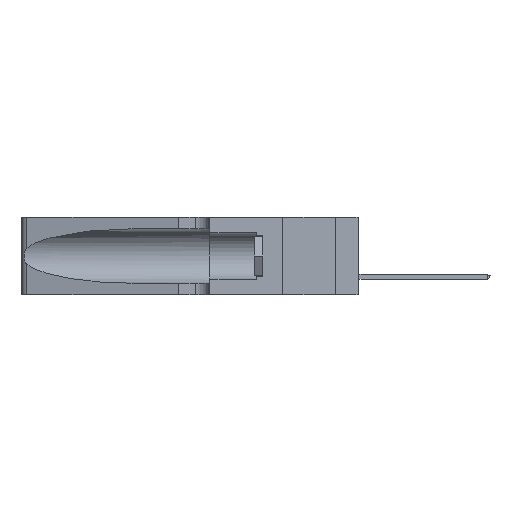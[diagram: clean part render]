
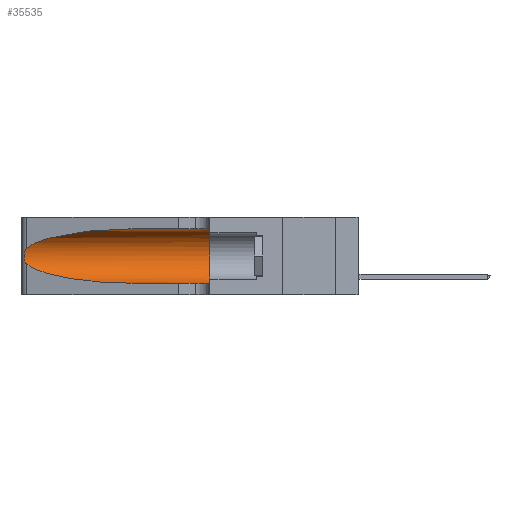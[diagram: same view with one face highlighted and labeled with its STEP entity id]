
A CAD part, left-side view. The second image highlights one B-rep face of the part: STEP entity #35535.
In plain terms, the highlighted cylindrical face has radius 3.308 mm (diameter 6.617 mm), a partial arc.
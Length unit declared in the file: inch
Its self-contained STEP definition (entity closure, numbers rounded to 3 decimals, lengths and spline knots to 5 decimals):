
#2345 = CARTESIAN_POINT ( 'NONE',  ( 0.1305, 0.72297, 0.05475 ) ) ;
#2667 = ORIENTED_EDGE ( 'NONE', *, *, #5160, .T. ) ;
#2709 = AXIS2_PLACEMENT_3D ( 'NONE', #33902, #11928, #28743 ) ;
#3378 = EDGE_LOOP ( 'NONE', ( #2667, #14993, #24889, #30679, #30256, #20336 ) ) ;
#3844 = CARTESIAN_POINT ( 'NONE',  ( 0.25487, 1.22718, 0.22369 ) ) ;
#3868 = CARTESIAN_POINT ( 'NONE',  ( 0.2373, 1.15595, 0.28018 ) ) ;
#4528 = VERTEX_POINT ( 'NONE', #35664 ) ;
#5133 = CARTESIAN_POINT ( 'NONE',  ( 0.1305, 0.72297, 0.31525 ) ) ;
#5160 = EDGE_CURVE ( 'NONE', #8227, #20518, #6681, .T. ) ;
#5359 = CARTESIAN_POINT ( 'NONE',  ( 0.1305, 0.35, 0.185 ) ) ;
#6681 =( BOUNDED_CURVE ( )  B_SPLINE_CURVE ( 3, ( #5133, #31014, #3868, #28514 ),
 .UNSPECIFIED., .F., .T. ) 
 B_SPLINE_CURVE_WITH_KNOTS ( ( 4, 4 ),
 ( 1.5708, 2.84003 ),
 .UNSPECIFIED. ) 
 CURVE ( )  GEOMETRIC_REPRESENTATION_ITEM ( )  RATIONAL_B_SPLINE_CURVE ( ( 1., 0.87, 0.87, 1. ) ) 
 REPRESENTATION_ITEM ( '' )  );
#7205 = CARTESIAN_POINT ( 'NONE',  ( 0.25639, 1.23184, 0.21858 ) ) ;
#7455 = CARTESIAN_POINT ( 'NONE',  ( 0.25487, 1.22718, 0.14631 ) ) ;
#7989 = CARTESIAN_POINT ( 'NONE',  ( 0.18966, 0.96281, 0.05475 ) ) ;
#8227 = VERTEX_POINT ( 'NONE', #12474 ) ;
#9101 = EDGE_CURVE ( 'NONE', #24137, #17811, #9318, .T. ) ;
#9318 =( BOUNDED_CURVE ( )  B_SPLINE_CURVE ( 3, ( #13550, #18970, #7989, #2345 ),
 .UNSPECIFIED., .F., .F. ) 
 B_SPLINE_CURVE_WITH_KNOTS ( ( 4, 4 ),
 ( 3.44316, 4.71239 ),
 .UNSPECIFIED. ) 
 CURVE ( )  GEOMETRIC_REPRESENTATION_ITEM ( )  RATIONAL_B_SPLINE_CURVE ( ( 1., 0.87, 0.87, 1. ) ) 
 REPRESENTATION_ITEM ( '' )  );
#9974 = CARTESIAN_POINT ( 'NONE',  ( 0.25789, 1.23486, 0.15765 ) ) ;
#11136 = AXIS2_PLACEMENT_3D ( 'NONE', #5359, #24618, #32941 ) ;
#11262 = CARTESIAN_POINT ( 'NONE',  ( 0.1305, 1.61858, 0.31525 ) ) ;
#11928 = DIRECTION ( 'NONE',  ( 0., -1., 0. ) ) ;
#12474 = CARTESIAN_POINT ( 'NONE',  ( 0.1305, 0.72297, 0.31525 ) ) ;
#13550 = CARTESIAN_POINT ( 'NONE',  ( 0.25487, 1.22718, 0.14631 ) ) ;
#14307 = FACE_OUTER_BOUND ( 'NONE', #3378, .T. ) ;
#14993 = ORIENTED_EDGE ( 'NONE', *, *, #34136, .T. ) ;
#15282 = CARTESIAN_POINT ( 'NONE',  ( 0.25787, 1.23484, 0.2124 ) ) ;
#15408 = CARTESIAN_POINT ( 'NONE',  ( 0.26075, 1.23896, 0.178 ) ) ;
#16091 = EDGE_CURVE ( 'NONE', #4528, #29876, #18589, .T. ) ;
#16310 = CARTESIAN_POINT ( 'NONE',  ( 0.25487, 1.22718, 0.14631 ) ) ;
#17081 = LINE ( 'NONE', #22098, #18355 ) ;
#17811 = VERTEX_POINT ( 'NONE', #28584 ) ;
#17942 = CARTESIAN_POINT ( 'NONE',  ( 0.25854, 1.2359, 0.20912 ) ) ;
#18355 = VECTOR ( 'NONE', #33048, 39.37008 ) ;
#18589 = CIRCLE ( 'NONE', #11136, 0.13025 ) ;
#18970 = CARTESIAN_POINT ( 'NONE',  ( 0.2373, 1.15595, 0.08982 ) ) ;
#19556 = VECTOR ( 'NONE', #19923, 39.37008 ) ;
#19923 = DIRECTION ( 'NONE',  ( 0., -1., 0. ) ) ;
#20336 = ORIENTED_EDGE ( 'NONE', *, *, #20964, .F. ) ;
#20518 = VERTEX_POINT ( 'NONE', #3844 ) ;
#20623 = CARTESIAN_POINT ( 'NONE',  ( 0.25555, 1.22994, 0.2215 ) ) ;
#20749 = CARTESIAN_POINT ( 'NONE',  ( 0.26018, 1.23835, 0.19895 ) ) ;
#20964 = EDGE_CURVE ( 'NONE', #8227, #4528, #31642, .T. ) ;
#20988 = CARTESIAN_POINT ( 'NONE',  ( 0.26017, 1.23833, 0.17102 ) ) ;
#22098 = CARTESIAN_POINT ( 'NONE',  ( 0.1305, 1.61858, 0.05475 ) ) ;
#22159 = CARTESIAN_POINT ( 'NONE',  ( 0.1305, 0.35, 0.05475 ) ) ;
#24137 = VERTEX_POINT ( 'NONE', #16310 ) ;
#24618 = DIRECTION ( 'NONE',  ( 0., 1., 0. ) ) ;
#24668 = CYLINDRICAL_SURFACE ( 'NONE', #2709, 0.13025 ) ;
#24889 = ORIENTED_EDGE ( 'NONE', *, *, #9101, .T. ) ;
#26338 = EDGE_CURVE ( 'NONE', #17811, #29876, #17081, .T. ) ;
#26525 = CARTESIAN_POINT ( 'NONE',  ( 0.25856, 1.23593, 0.16098 ) ) ;
#28514 = CARTESIAN_POINT ( 'NONE',  ( 0.25487, 1.22718, 0.22369 ) ) ;
#28584 = CARTESIAN_POINT ( 'NONE',  ( 0.1305, 0.72297, 0.05475 ) ) ;
#28743 = DIRECTION ( 'NONE',  ( 0., 0., -1. ) ) ;
#29876 = VERTEX_POINT ( 'NONE', #22159 ) ;
#30256 = ORIENTED_EDGE ( 'NONE', *, *, #16091, .F. ) ;
#30679 = ORIENTED_EDGE ( 'NONE', *, *, #26338, .T. ) ;
#31014 = CARTESIAN_POINT ( 'NONE',  ( 0.18966, 0.96281, 0.31525 ) ) ;
#31224 = B_SPLINE_CURVE_WITH_KNOTS ( 'NONE', 3,
 ( #31928, #20623, #7205, #15282, #17942, #20749, #31691, #15408, #20988, #26525, #9974, #32052, #32163, #7455 ),
 .UNSPECIFIED., .F., .F.,
 ( 4, 2, 2, 2, 2, 2, 4 ),
 ( 0., 0.00027, 0.00053, 0.00107, 0.0016, 0.00187, 0.00214 ),
 .UNSPECIFIED. ) ;
#31642 = LINE ( 'NONE', #11262, #19556 ) ;
#31691 = CARTESIAN_POINT ( 'NONE',  ( 0.26075, 1.23896, 0.19203 ) ) ;
#31928 = CARTESIAN_POINT ( 'NONE',  ( 0.25487, 1.22718, 0.22369 ) ) ;
#32052 = CARTESIAN_POINT ( 'NONE',  ( 0.25639, 1.23186, 0.15144 ) ) ;
#32163 = CARTESIAN_POINT ( 'NONE',  ( 0.25555, 1.22993, 0.14849 ) ) ;
#32941 = DIRECTION ( 'NONE',  ( 0., 0., 1. ) ) ;
#33048 = DIRECTION ( 'NONE',  ( 0., -1., 0. ) ) ;
#33902 = CARTESIAN_POINT ( 'NONE',  ( 0.1305, 1.61858, 0.185 ) ) ;
#34136 = EDGE_CURVE ( 'NONE', #20518, #24137, #31224, .T. ) ;
#35535 = ADVANCED_FACE ( 'NONE', ( #14307 ), #24668, .F. ) ;
#35664 = CARTESIAN_POINT ( 'NONE',  ( 0.1305, 0.35, 0.31525 ) ) ;
